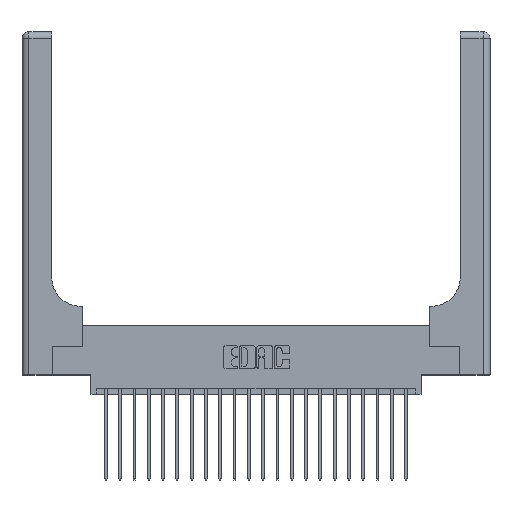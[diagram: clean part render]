
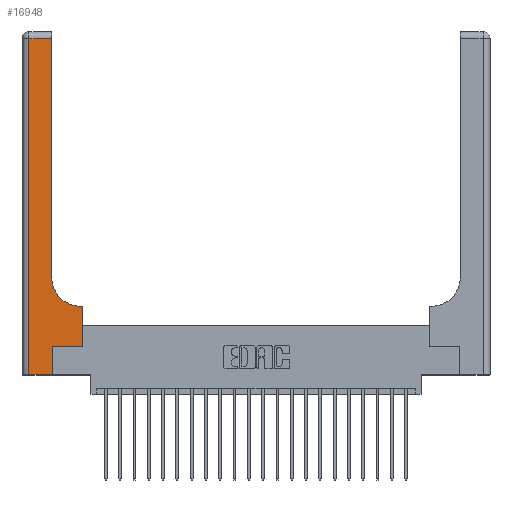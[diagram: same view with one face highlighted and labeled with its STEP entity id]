
A CAD part, top view. The second image highlights one B-rep face of the part: STEP entity #16948.
In plain terms, the highlighted planar face has unit normal (0, 0, 1).
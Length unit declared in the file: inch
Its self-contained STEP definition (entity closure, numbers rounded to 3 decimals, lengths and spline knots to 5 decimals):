
#482 = EDGE_CURVE ( 'NONE', #14374, #21456, #2418, .T. ) ;
#974 = LINE ( 'NONE', #15161, #13821 ) ;
#2090 = LINE ( 'NONE', #3268, #20000 ) ;
#2418 = LINE ( 'NONE', #4724, #20335 ) ;
#2534 = CARTESIAN_POINT ( 'NONE',  ( 0.51, 0.85, 0.37 ) ) ;
#2955 = DIRECTION ( 'NONE',  ( -1., 0., 0. ) ) ;
#3080 = EDGE_CURVE ( 'NONE', #18849, #5858, #4571, .T. ) ;
#3268 = CARTESIAN_POINT ( 'NONE',  ( 0.26, 3., 0.37 ) ) ;
#3478 = DIRECTION ( 'NONE',  ( 1., 0., 0. ) ) ;
#3836 = ORIENTED_EDGE ( 'NONE', *, *, #3977, .T. ) ;
#3883 = DIRECTION ( 'NONE',  ( 0., -1., 0. ) ) ;
#3944 = CARTESIAN_POINT ( 'NONE',  ( 0.528, 0.25, 0.37 ) ) ;
#3977 = EDGE_CURVE ( 'NONE', #4271, #14374, #974, .T. ) ;
#4225 = CARTESIAN_POINT ( 'NONE',  ( 0.528, 0.25, 0.37 ) ) ;
#4271 = VERTEX_POINT ( 'NONE', #7165 ) ;
#4308 = DIRECTION ( 'NONE',  ( 1., 0., 0. ) ) ;
#4571 = LINE ( 'NONE', #10214, #17927 ) ;
#4724 = CARTESIAN_POINT ( 'NONE',  ( 0.06, 3., 0.37 ) ) ;
#4862 = CARTESIAN_POINT ( 'NONE',  ( 0., 3., 0.37 ) ) ;
#5030 = CARTESIAN_POINT ( 'NONE',  ( 0., 0., 0.37 ) ) ;
#5735 = ORIENTED_EDGE ( 'NONE', *, *, #21789, .T. ) ;
#5768 = LINE ( 'NONE', #5030, #9309 ) ;
#5787 = EDGE_CURVE ( 'NONE', #20987, #18849, #12923, .T. ) ;
#5858 = VERTEX_POINT ( 'NONE', #11145 ) ;
#6401 = AXIS2_PLACEMENT_3D ( 'NONE', #4862, #22137, #11896 ) ;
#6402 = CARTESIAN_POINT ( 'NONE',  ( 0.528, 0.6, 0.37 ) ) ;
#6783 = DIRECTION ( 'NONE',  ( 1., 0., 0. ) ) ;
#7165 = CARTESIAN_POINT ( 'NONE',  ( 0.26, 2.94, 0.37 ) ) ;
#7192 = DIRECTION ( 'NONE',  ( 0., 1., 0. ) ) ;
#8367 = PLANE ( 'NONE',  #6401 ) ;
#8457 = EDGE_CURVE ( 'NONE', #21456, #18913, #5768, .T. ) ;
#8554 = ORIENTED_EDGE ( 'NONE', *, *, #482, .T. ) ;
#8557 = EDGE_CURVE ( 'NONE', #17803, #20987, #12320, .T. ) ;
#9087 = ORIENTED_EDGE ( 'NONE', *, *, #8457, .T. ) ;
#9309 = VECTOR ( 'NONE', #6783, 39.37008 ) ;
#9637 = ORIENTED_EDGE ( 'NONE', *, *, #13272, .T. ) ;
#10214 = CARTESIAN_POINT ( 'NONE',  ( 0.26, 0.6, 0.37 ) ) ;
#10443 = ORIENTED_EDGE ( 'NONE', *, *, #8557, .T. ) ;
#10783 = CARTESIAN_POINT ( 'NONE',  ( 0.265, 0.25, 0.37 ) ) ;
#11145 = CARTESIAN_POINT ( 'NONE',  ( 0.51, 0.6, 0.37 ) ) ;
#11615 = FACE_OUTER_BOUND ( 'NONE', #14510, .T. ) ;
#11656 = VECTOR ( 'NONE', #7192, 39.37008 ) ;
#11896 = DIRECTION ( 'NONE',  ( -1., 0., 0. ) ) ;
#11940 = VERTEX_POINT ( 'NONE', #15790 ) ;
#12186 = CARTESIAN_POINT ( 'NONE',  ( 0.06, 2.94, 0.37 ) ) ;
#12199 = LINE ( 'NONE', #19325, #11656 ) ;
#12320 = LINE ( 'NONE', #12654, #21402 ) ;
#12654 = CARTESIAN_POINT ( 'NONE',  ( 0.265, 0.25, 0.37 ) ) ;
#12923 = LINE ( 'NONE', #3944, #22016 ) ;
#13218 = ORIENTED_EDGE ( 'NONE', *, *, #5787, .T. ) ;
#13272 = EDGE_CURVE ( 'NONE', #18913, #17803, #12199, .T. ) ;
#13734 = DIRECTION ( 'NONE',  ( 0., 1., 0. ) ) ;
#13821 = VECTOR ( 'NONE', #2955, 39.37008 ) ;
#14005 = ORIENTED_EDGE ( 'NONE', *, *, #3080, .T. ) ;
#14330 = AXIS2_PLACEMENT_3D ( 'NONE', #2534, #14754, #4308 ) ;
#14374 = VERTEX_POINT ( 'NONE', #12186 ) ;
#14510 = EDGE_LOOP ( 'NONE', ( #17810, #3836, #8554, #9087, #9637, #10443, #13218, #14005, #5735 ) ) ;
#14754 = DIRECTION ( 'NONE',  ( 0., 0., -1. ) ) ;
#15161 = CARTESIAN_POINT ( 'NONE',  ( 0., 2.94, 0.37 ) ) ;
#15790 = CARTESIAN_POINT ( 'NONE',  ( 0.26, 0.85, 0.37 ) ) ;
#16948 = ADVANCED_FACE ( 'NONE', ( #11615 ), #8367, .F. ) ;
#17353 = CARTESIAN_POINT ( 'NONE',  ( 0.06, 0., 0.37 ) ) ;
#17803 = VERTEX_POINT ( 'NONE', #10783 ) ;
#17810 = ORIENTED_EDGE ( 'NONE', *, *, #18296, .T. ) ;
#17927 = VECTOR ( 'NONE', #22203, 39.37008 ) ;
#18296 = EDGE_CURVE ( 'NONE', #11940, #4271, #2090, .T. ) ;
#18704 = CARTESIAN_POINT ( 'NONE',  ( 0.265, 0., 0.37 ) ) ;
#18849 = VERTEX_POINT ( 'NONE', #6402 ) ;
#18913 = VERTEX_POINT ( 'NONE', #18704 ) ;
#19325 = CARTESIAN_POINT ( 'NONE',  ( 0.265, 0., 0.37 ) ) ;
#19593 = DIRECTION ( 'NONE',  ( 0., 1., 0. ) ) ;
#20000 = VECTOR ( 'NONE', #13734, 39.37008 ) ;
#20335 = VECTOR ( 'NONE', #3883, 39.37008 ) ;
#20635 = CIRCLE ( 'NONE', #14330, 0.25 ) ;
#20987 = VERTEX_POINT ( 'NONE', #4225 ) ;
#21402 = VECTOR ( 'NONE', #3478, 39.37008 ) ;
#21456 = VERTEX_POINT ( 'NONE', #17353 ) ;
#21789 = EDGE_CURVE ( 'NONE', #5858, #11940, #20635, .T. ) ;
#22016 = VECTOR ( 'NONE', #19593, 39.37008 ) ;
#22137 = DIRECTION ( 'NONE',  ( 0., 0., -1. ) ) ;
#22203 = DIRECTION ( 'NONE',  ( -1., 0., 0. ) ) ;
